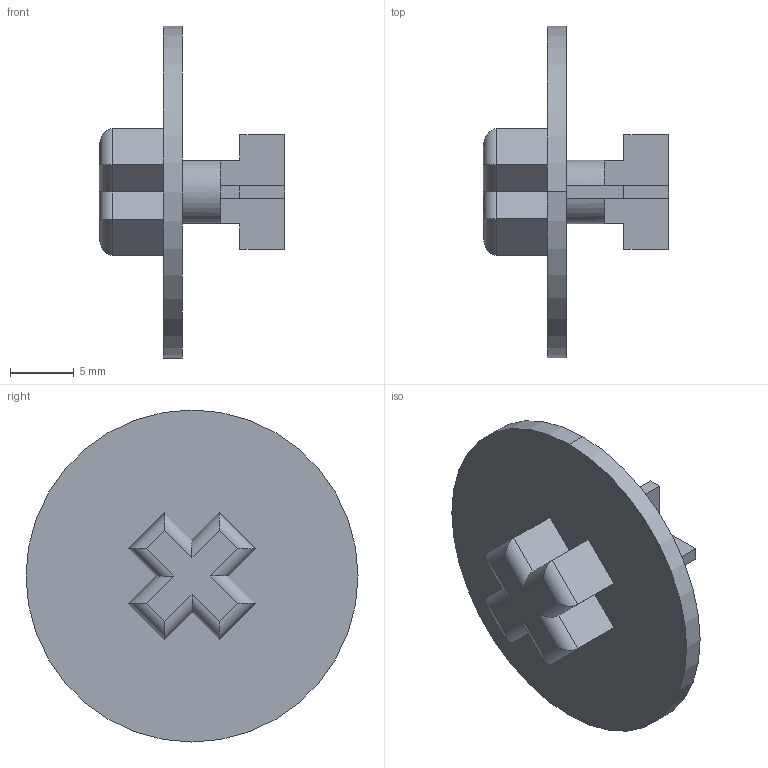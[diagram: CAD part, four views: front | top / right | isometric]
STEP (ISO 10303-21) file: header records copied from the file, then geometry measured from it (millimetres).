
FILE_DESCRIPTION (( 'STEP AP203' ), '1' );
FILE_NAME ('back_plate.STEP', '2013-07-12T02:41:59', ( '' ), ( '' ), 'SwSTEP 2.0', 'SolidWorks 2012', '' );
FILE_SCHEMA (( 'CONFIG_CONTROL_DESIGN' ));
Length unit declared in the file: millimetre
Products named in the file (1): back_plate
Bounding box: 14.5 x 26 x 26 mm (x, y, z)
Volume: 1240.2 mm3; surface area: 1586.4 mm2
Topology: 1 solids, 1 shells, 60 faces, 150 edges, 94 vertices
Faces by surface type: plane 44, cylinder 16
Entity records: 1821 total; most frequent: CARTESIAN_POINT 341, ORIENTED_EDGE 300, DIRECTION 274, EDGE_CURVE 150, VECTOR 124, LINE 124, VERTEX_POINT 94, AXIS2_PLACEMENT_3D 75
